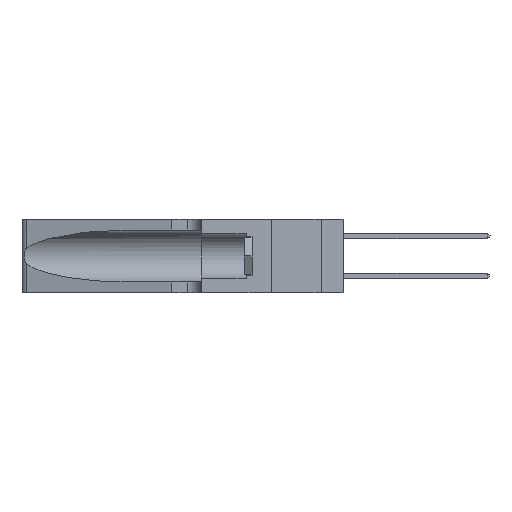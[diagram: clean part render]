
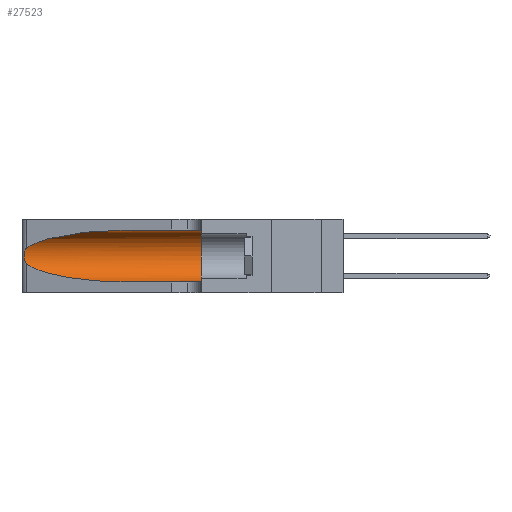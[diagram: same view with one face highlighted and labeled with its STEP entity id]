
A CAD part, left-side view. The second image highlights one B-rep face of the part: STEP entity #27523.
In plain terms, the highlighted cylindrical face has radius 3.308 mm (diameter 6.617 mm), a partial arc.
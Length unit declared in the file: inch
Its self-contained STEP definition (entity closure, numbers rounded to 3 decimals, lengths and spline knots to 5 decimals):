
#124 = DIRECTION ( 'NONE',  ( 0., 1., 0. ) ) ;
#522 = CARTESIAN_POINT ( 'NONE',  ( 0.26017, 1.23833, 0.17102 ) ) ;
#674 = CARTESIAN_POINT ( 'NONE',  ( 0.26075, 1.23896, 0.178 ) ) ;
#1770 = CARTESIAN_POINT ( 'NONE',  ( 0.25787, 1.23484, 0.2124 ) ) ;
#3029 = CARTESIAN_POINT ( 'NONE',  ( 0.1305, 1.61858, 0.05475 ) ) ;
#4864 = EDGE_CURVE ( 'NONE', #12097, #11912, #6760, .T. ) ;
#5084 = EDGE_CURVE ( 'NONE', #21207, #20813, #41048, .T. ) ;
#5269 = CARTESIAN_POINT ( 'NONE',  ( 0.25639, 1.23184, 0.21858 ) ) ;
#6306 = CARTESIAN_POINT ( 'NONE',  ( 0.1305, 0.35, 0.185 ) ) ;
#6355 = CARTESIAN_POINT ( 'NONE',  ( 0.26018, 1.23835, 0.19895 ) ) ;
#6380 = DIRECTION ( 'NONE',  ( 0., -1., 0. ) ) ;
#6642 = ORIENTED_EDGE ( 'NONE', *, *, #5084, .T. ) ;
#6752 = CARTESIAN_POINT ( 'NONE',  ( 0.25856, 1.23593, 0.16098 ) ) ;
#6760 =( BOUNDED_CURVE ( )  B_SPLINE_CURVE ( 3, ( #19729, #14086, #19510, #29443 ),
 .UNSPECIFIED., .F., .F. ) 
 B_SPLINE_CURVE_WITH_KNOTS ( ( 4, 4 ),
 ( 1.5708, 2.84003 ),
 .UNSPECIFIED. ) 
 CURVE ( )  GEOMETRIC_REPRESENTATION_ITEM ( )  RATIONAL_B_SPLINE_CURVE ( ( 1., 0.87, 0.87, 1. ) ) 
 REPRESENTATION_ITEM ( '' )  );
#8882 = CARTESIAN_POINT ( 'NONE',  ( 0.1305, 0.72297, 0.05475 ) ) ;
#9940 = ORIENTED_EDGE ( 'NONE', *, *, #19176, .T. ) ;
#10781 = ORIENTED_EDGE ( 'NONE', *, *, #32199, .F. ) ;
#11639 = ORIENTED_EDGE ( 'NONE', *, *, #4864, .T. ) ;
#11912 = VERTEX_POINT ( 'NONE', #16055 ) ;
#12097 = VERTEX_POINT ( 'NONE', #34414 ) ;
#12172 = AXIS2_PLACEMENT_3D ( 'NONE', #6306, #124, #13053 ) ;
#12643 = DIRECTION ( 'NONE',  ( 0., -1., 0. ) ) ;
#12716 = CARTESIAN_POINT ( 'NONE',  ( 0.18966, 0.96281, 0.05475 ) ) ;
#12986 = CARTESIAN_POINT ( 'NONE',  ( 0.25487, 1.22718, 0.14631 ) ) ;
#13053 = DIRECTION ( 'NONE',  ( 0., 0., 1. ) ) ;
#14086 = CARTESIAN_POINT ( 'NONE',  ( 0.18966, 0.96281, 0.31525 ) ) ;
#14868 = CARTESIAN_POINT ( 'NONE',  ( 0.25487, 1.22718, 0.22369 ) ) ;
#15976 = EDGE_LOOP ( 'NONE', ( #11639, #16882, #6642, #9940, #29175, #10781 ) ) ;
#16055 = CARTESIAN_POINT ( 'NONE',  ( 0.25487, 1.22718, 0.22369 ) ) ;
#16099 = CARTESIAN_POINT ( 'NONE',  ( 0.2373, 1.15595, 0.08982 ) ) ;
#16618 = FACE_OUTER_BOUND ( 'NONE', #15976, .T. ) ;
#16882 = ORIENTED_EDGE ( 'NONE', *, *, #26648, .T. ) ;
#19176 = EDGE_CURVE ( 'NONE', #20813, #19817, #33765, .T. ) ;
#19210 = CARTESIAN_POINT ( 'NONE',  ( 0.1305, 0.35, 0.05475 ) ) ;
#19510 = CARTESIAN_POINT ( 'NONE',  ( 0.2373, 1.15595, 0.28018 ) ) ;
#19729 = CARTESIAN_POINT ( 'NONE',  ( 0.1305, 0.72297, 0.31525 ) ) ;
#19733 = CARTESIAN_POINT ( 'NONE',  ( 0.25639, 1.23186, 0.15144 ) ) ;
#19817 = VERTEX_POINT ( 'NONE', #19210 ) ;
#19870 = CARTESIAN_POINT ( 'NONE',  ( 0.26075, 1.23896, 0.19203 ) ) ;
#20813 = VERTEX_POINT ( 'NONE', #8882 ) ;
#21207 = VERTEX_POINT ( 'NONE', #37935 ) ;
#21223 = CARTESIAN_POINT ( 'NONE',  ( 0.25854, 1.2359, 0.20912 ) ) ;
#22005 = LINE ( 'NONE', #26911, #29026 ) ;
#22116 = CARTESIAN_POINT ( 'NONE',  ( 0.1305, 1.61858, 0.185 ) ) ;
#23084 = CARTESIAN_POINT ( 'NONE',  ( 0.25555, 1.22993, 0.14849 ) ) ;
#26299 = CARTESIAN_POINT ( 'NONE',  ( 0.25487, 1.22718, 0.14631 ) ) ;
#26648 = EDGE_CURVE ( 'NONE', #11912, #21207, #33867, .T. ) ;
#26911 = CARTESIAN_POINT ( 'NONE',  ( 0.1305, 1.61858, 0.31525 ) ) ;
#27523 = ADVANCED_FACE ( 'NONE', ( #16618 ), #29218, .F. ) ;
#29026 = VECTOR ( 'NONE', #30285, 39.37008 ) ;
#29175 = ORIENTED_EDGE ( 'NONE', *, *, #41453, .F. ) ;
#29218 = CYLINDRICAL_SURFACE ( 'NONE', #39779, 0.13025 ) ;
#29276 = CARTESIAN_POINT ( 'NONE',  ( 0.25789, 1.23486, 0.15765 ) ) ;
#29443 = CARTESIAN_POINT ( 'NONE',  ( 0.25487, 1.22718, 0.22369 ) ) ;
#29952 = CARTESIAN_POINT ( 'NONE',  ( 0.1305, 0.35, 0.31525 ) ) ;
#30244 = VECTOR ( 'NONE', #6380, 39.37008 ) ;
#30285 = DIRECTION ( 'NONE',  ( 0., -1., 0. ) ) ;
#30939 = CIRCLE ( 'NONE', #12172, 0.13025 ) ;
#32199 = EDGE_CURVE ( 'NONE', #12097, #36304, #22005, .T. ) ;
#33765 = LINE ( 'NONE', #3029, #30244 ) ;
#33867 = B_SPLINE_CURVE_WITH_KNOTS ( 'NONE', 3,
 ( #14868, #37045, #5269, #1770, #21223, #6355, #19870, #674, #522, #6752, #29276, #19733, #23084, #26299 ),
 .UNSPECIFIED., .F., .F.,
 ( 4, 2, 2, 2, 2, 2, 4 ),
 ( 0., 0.00027, 0.00053, 0.00107, 0.0016, 0.00187, 0.00214 ),
 .UNSPECIFIED. ) ;
#34414 = CARTESIAN_POINT ( 'NONE',  ( 0.1305, 0.72297, 0.31525 ) ) ;
#35179 = DIRECTION ( 'NONE',  ( 0., 0., -1. ) ) ;
#36304 = VERTEX_POINT ( 'NONE', #29952 ) ;
#37045 = CARTESIAN_POINT ( 'NONE',  ( 0.25555, 1.22994, 0.2215 ) ) ;
#37935 = CARTESIAN_POINT ( 'NONE',  ( 0.25487, 1.22718, 0.14631 ) ) ;
#38557 = CARTESIAN_POINT ( 'NONE',  ( 0.1305, 0.72297, 0.05475 ) ) ;
#39779 = AXIS2_PLACEMENT_3D ( 'NONE', #22116, #12643, #35179 ) ;
#41048 =( BOUNDED_CURVE ( )  B_SPLINE_CURVE ( 3, ( #12986, #16099, #12716, #38557 ),
 .UNSPECIFIED., .F., .F. ) 
 B_SPLINE_CURVE_WITH_KNOTS ( ( 4, 4 ),
 ( 3.44316, 4.71239 ),
 .UNSPECIFIED. ) 
 CURVE ( )  GEOMETRIC_REPRESENTATION_ITEM ( )  RATIONAL_B_SPLINE_CURVE ( ( 1., 0.87, 0.87, 1. ) ) 
 REPRESENTATION_ITEM ( '' )  );
#41453 = EDGE_CURVE ( 'NONE', #36304, #19817, #30939, .T. ) ;
